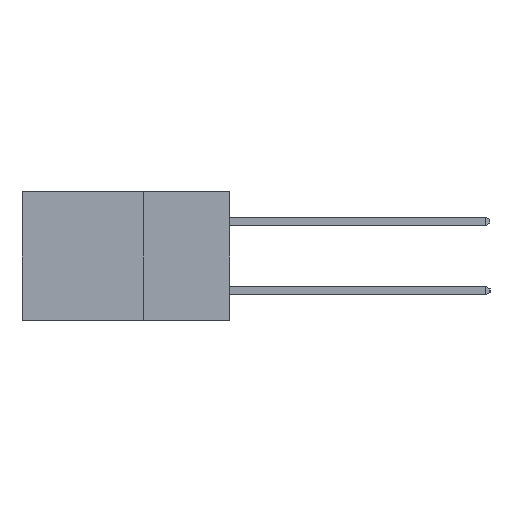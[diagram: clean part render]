
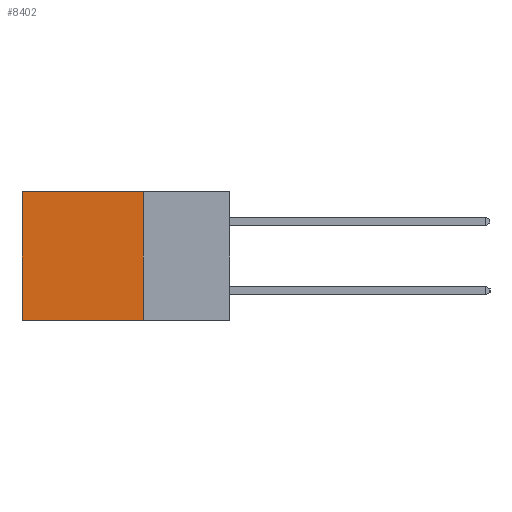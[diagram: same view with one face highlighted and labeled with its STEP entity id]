
A CAD part, left-side view. The second image highlights one B-rep face of the part: STEP entity #8402.
In plain terms, the highlighted planar face has unit normal (-1, 0, 0).
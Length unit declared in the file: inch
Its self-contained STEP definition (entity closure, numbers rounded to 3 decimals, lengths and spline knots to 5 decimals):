
#738 = CARTESIAN_POINT ( 'NONE',  ( 0.2615, 0.25, -0.37 ) ) ;
#2367 = DIRECTION ( 'NONE',  ( 0., 1., 0. ) ) ;
#2428 = VERTEX_POINT ( 'NONE', #19757 ) ;
#2970 = ORIENTED_EDGE ( 'NONE', *, *, #7508, .F. ) ;
#3089 = LINE ( 'NONE', #738, #19233 ) ;
#3105 = ORIENTED_EDGE ( 'NONE', *, *, #13878, .F. ) ;
#3953 = ORIENTED_EDGE ( 'NONE', *, *, #13500, .T. ) ;
#4721 = CARTESIAN_POINT ( 'NONE',  ( 0.2615, 0.6, -0.37 ) ) ;
#6042 = LINE ( 'NONE', #14834, #14652 ) ;
#6078 = VERTEX_POINT ( 'NONE', #7556 ) ;
#7508 = EDGE_CURVE ( 'NONE', #19420, #6078, #6042, .T. ) ;
#7556 = CARTESIAN_POINT ( 'NONE',  ( 0.2615, 0.25, -0.37 ) ) ;
#8158 = CARTESIAN_POINT ( 'NONE',  ( 0.2615, 0.25, 0. ) ) ;
#8402 = ADVANCED_FACE ( 'NONE', ( #20451 ), #14983, .F. ) ;
#9662 = VERTEX_POINT ( 'NONE', #11239 ) ;
#11239 = CARTESIAN_POINT ( 'NONE',  ( 0.2615, 0.6, 0. ) ) ;
#13037 = DIRECTION ( 'NONE',  ( 0., 1., 0. ) ) ;
#13408 = AXIS2_PLACEMENT_3D ( 'NONE', #15130, #14932, #14888 ) ;
#13500 = EDGE_CURVE ( 'NONE', #9662, #2428, #18263, .T. ) ;
#13878 = EDGE_CURVE ( 'NONE', #6078, #2428, #3089, .T. ) ;
#14005 = VECTOR ( 'NONE', #14449, 39.37008 ) ;
#14057 = CARTESIAN_POINT ( 'NONE',  ( 0.2615, 0.25, 0. ) ) ;
#14432 = EDGE_LOOP ( 'NONE', ( #3953, #3105, #2970, #19149 ) ) ;
#14449 = DIRECTION ( 'NONE',  ( 0., 0., -1. ) ) ;
#14652 = VECTOR ( 'NONE', #14812, 39.37008 ) ;
#14812 = DIRECTION ( 'NONE',  ( 0., 0., -1. ) ) ;
#14834 = CARTESIAN_POINT ( 'NONE',  ( 0.2615, 0.25, -0.37 ) ) ;
#14888 = DIRECTION ( 'NONE',  ( 0., 0., -1. ) ) ;
#14932 = DIRECTION ( 'NONE',  ( 1., 0., 0. ) ) ;
#14983 = PLANE ( 'NONE',  #13408 ) ;
#15061 = EDGE_CURVE ( 'NONE', #19420, #9662, #16778, .T. ) ;
#15130 = CARTESIAN_POINT ( 'NONE',  ( 0.2615, 0.25, -0.37 ) ) ;
#16264 = VECTOR ( 'NONE', #13037, 39.37008 ) ;
#16778 = LINE ( 'NONE', #8158, #16264 ) ;
#18263 = LINE ( 'NONE', #4721, #14005 ) ;
#19149 = ORIENTED_EDGE ( 'NONE', *, *, #15061, .T. ) ;
#19233 = VECTOR ( 'NONE', #2367, 39.37008 ) ;
#19420 = VERTEX_POINT ( 'NONE', #14057 ) ;
#19757 = CARTESIAN_POINT ( 'NONE',  ( 0.2615, 0.6, -0.37 ) ) ;
#20451 = FACE_OUTER_BOUND ( 'NONE', #14432, .T. ) ;
